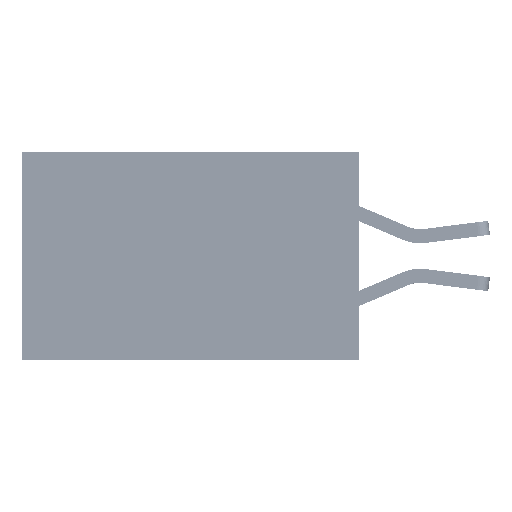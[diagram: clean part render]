
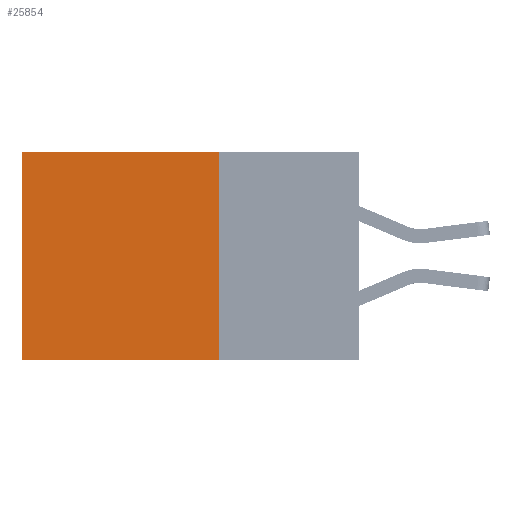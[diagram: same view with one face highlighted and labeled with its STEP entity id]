
A CAD part, left-side view. The second image highlights one B-rep face of the part: STEP entity #25854.
In plain terms, the highlighted planar face has unit normal (-1, 0, 0).
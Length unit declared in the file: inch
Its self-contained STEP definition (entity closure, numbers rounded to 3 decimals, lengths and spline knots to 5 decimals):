
#132 = FACE_OUTER_BOUND ( 'NONE', #5148, .T. ) ;
#523 = VERTEX_POINT ( 'NONE', #8824 ) ;
#1693 = DIRECTION ( 'NONE',  ( 0., 0., -1. ) ) ;
#3077 = CARTESIAN_POINT ( 'NONE',  ( 0.2875, 0.25, -0.37 ) ) ;
#3206 = CARTESIAN_POINT ( 'NONE',  ( 0.2875, 0.25, 0. ) ) ;
#3418 = CARTESIAN_POINT ( 'NONE',  ( 0.2875, 0.25, 0. ) ) ;
#4077 = LINE ( 'NONE', #6717, #26492 ) ;
#4126 = LINE ( 'NONE', #3077, #7702 ) ;
#5148 = EDGE_LOOP ( 'NONE', ( #9149, #10351, #12524, #35642 ) ) ;
#5577 = PLANE ( 'NONE',  #35401 ) ;
#6717 = CARTESIAN_POINT ( 'NONE',  ( 0.2875, 0.6, 0. ) ) ;
#7702 = VECTOR ( 'NONE', #9189, 39.37008 ) ;
#8824 = CARTESIAN_POINT ( 'NONE',  ( 0.2875, 0.25, -0.37 ) ) ;
#8867 = EDGE_CURVE ( 'NONE', #8963, #20911, #20185, .T. ) ;
#8963 = VERTEX_POINT ( 'NONE', #3418 ) ;
#9149 = ORIENTED_EDGE ( 'NONE', *, *, #18785, .T. ) ;
#9189 = DIRECTION ( 'NONE',  ( 0., 1., 0. ) ) ;
#10351 = ORIENTED_EDGE ( 'NONE', *, *, #29569, .F. ) ;
#11299 = DIRECTION ( 'NONE',  ( 0., 1., 0. ) ) ;
#11564 = DIRECTION ( 'NONE',  ( 0., 0., -1. ) ) ;
#12217 = DIRECTION ( 'NONE',  ( 0., 0., -1. ) ) ;
#12524 = ORIENTED_EDGE ( 'NONE', *, *, #15409, .F. ) ;
#12529 = VECTOR ( 'NONE', #11299, 39.37008 ) ;
#14336 = VERTEX_POINT ( 'NONE', #32008 ) ;
#14733 = DIRECTION ( 'NONE',  ( 1., 0., 0. ) ) ;
#15192 = CARTESIAN_POINT ( 'NONE',  ( 0.2875, 0.6, 0. ) ) ;
#15409 = EDGE_CURVE ( 'NONE', #8963, #523, #26050, .T. ) ;
#18785 = EDGE_CURVE ( 'NONE', #20911, #14336, #4077, .T. ) ;
#20185 = LINE ( 'NONE', #34453, #12529 ) ;
#20911 = VERTEX_POINT ( 'NONE', #15192 ) ;
#25854 = ADVANCED_FACE ( 'NONE', ( #132 ), #5577, .F. ) ;
#26050 = LINE ( 'NONE', #36338, #31904 ) ;
#26492 = VECTOR ( 'NONE', #12217, 39.37008 ) ;
#29569 = EDGE_CURVE ( 'NONE', #523, #14336, #4126, .T. ) ;
#31904 = VECTOR ( 'NONE', #1693, 39.37008 ) ;
#32008 = CARTESIAN_POINT ( 'NONE',  ( 0.2875, 0.6, -0.37 ) ) ;
#34453 = CARTESIAN_POINT ( 'NONE',  ( 0.2875, 0.25, 0. ) ) ;
#35401 = AXIS2_PLACEMENT_3D ( 'NONE', #3206, #14733, #11564 ) ;
#35642 = ORIENTED_EDGE ( 'NONE', *, *, #8867, .T. ) ;
#36338 = CARTESIAN_POINT ( 'NONE',  ( 0.2875, 0.25, 0. ) ) ;
